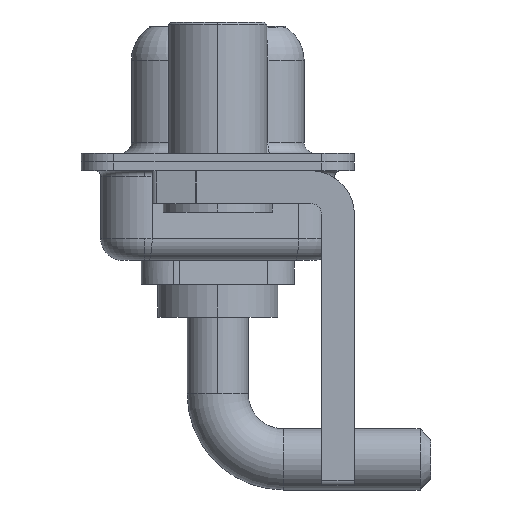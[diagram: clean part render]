
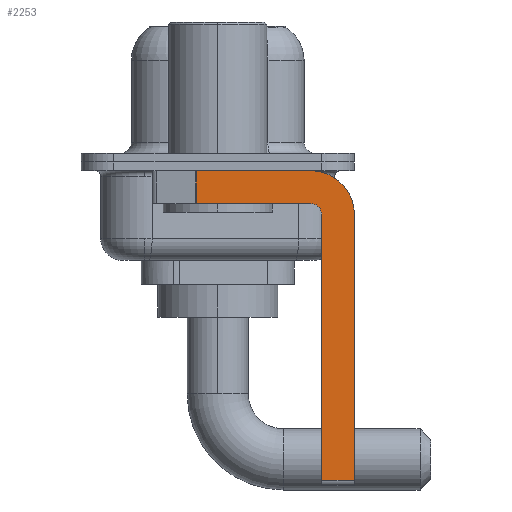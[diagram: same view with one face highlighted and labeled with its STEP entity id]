
A CAD part, left-side view. The second image highlights one B-rep face of the part: STEP entity #2253.
In plain terms, the highlighted planar face has unit normal (-1, 0, 0).
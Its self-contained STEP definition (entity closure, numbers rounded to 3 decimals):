
#216 = EDGE_LOOP ( 'NONE', ( #5971, #10110, #9486, #14276, #6099, #7282, #8405, #11327 ) ) ;
#619 = CARTESIAN_POINT ( 'NONE',  ( -2.9, 3., -0.4 ) ) ;
#848 = VERTEX_POINT ( 'NONE', #3708 ) ;
#1447 = LINE ( 'NONE', #4755, #10010 ) ;
#1519 = VECTOR ( 'NONE', #13532, 1000. ) ;
#1612 = VECTOR ( 'NONE', #6368, 1000. ) ;
#1747 = LINE ( 'NONE', #619, #13849 ) ;
#1781 = CARTESIAN_POINT ( 'NONE',  ( -2.9, -6.25, -2.4 ) ) ;
#2015 = CIRCLE ( 'NONE', #3934, 2. ) ;
#2098 = LINE ( 'NONE', #12490, #3447 ) ;
#2253 = ADVANCED_FACE ( 'NONE', ( #9279 ), #13863, .F. ) ;
#3018 = CARTESIAN_POINT ( 'NONE',  ( -2.9, -6.25, -14.55 ) ) ;
#3193 = CARTESIAN_POINT ( 'NONE',  ( -2.9, -4.25, -2.4 ) ) ;
#3383 = CARTESIAN_POINT ( 'NONE',  ( -2.9, 0.978, -1.9 ) ) ;
#3447 = VECTOR ( 'NONE', #7899, 1000. ) ;
#3708 = CARTESIAN_POINT ( 'NONE',  ( -2.9, 0.978, -0.4 ) ) ;
#3718 = VERTEX_POINT ( 'NONE', #3018 ) ;
#3934 = AXIS2_PLACEMENT_3D ( 'NONE', #7556, #10956, #8694 ) ;
#4465 = DIRECTION ( 'NONE',  ( 0., 0., 1. ) ) ;
#4477 = EDGE_CURVE ( 'NONE', #10130, #3718, #10084, .T. ) ;
#4755 = CARTESIAN_POINT ( 'NONE',  ( -2.9, -4.75, -14.8 ) ) ;
#4839 = AXIS2_PLACEMENT_3D ( 'NONE', #6173, #5333, #7453 ) ;
#5162 = LINE ( 'NONE', #1781, #1612 ) ;
#5333 = DIRECTION ( 'NONE',  ( 1., 0., 0. ) ) ;
#5971 = ORIENTED_EDGE ( 'NONE', *, *, #13015, .F. ) ;
#6003 = EDGE_CURVE ( 'NONE', #12529, #3718, #5162, .T. ) ;
#6099 = ORIENTED_EDGE ( 'NONE', *, *, #12725, .F. ) ;
#6173 = CARTESIAN_POINT ( 'NONE',  ( -2.9, -4.25, -2.4 ) ) ;
#6368 = DIRECTION ( 'NONE',  ( 0., 0., -1. ) ) ;
#6545 = VERTEX_POINT ( 'NONE', #14383 ) ;
#7081 = AXIS2_PLACEMENT_3D ( 'NONE', #3193, #11256, #4465 ) ;
#7282 = ORIENTED_EDGE ( 'NONE', *, *, #4477, .T. ) ;
#7453 = DIRECTION ( 'NONE',  ( 0., 0., -1. ) ) ;
#7537 = VERTEX_POINT ( 'NONE', #13275 ) ;
#7556 = CARTESIAN_POINT ( 'NONE',  ( -2.9, -4.25, -2.4 ) ) ;
#7889 = VERTEX_POINT ( 'NONE', #9103 ) ;
#7899 = DIRECTION ( 'NONE',  ( 0., 1., 0. ) ) ;
#8007 = EDGE_CURVE ( 'NONE', #7889, #8033, #2098, .T. ) ;
#8033 = VERTEX_POINT ( 'NONE', #3383 ) ;
#8301 = DIRECTION ( 'NONE',  ( 0., 0., 1. ) ) ;
#8405 = ORIENTED_EDGE ( 'NONE', *, *, #6003, .F. ) ;
#8694 = DIRECTION ( 'NONE',  ( 0., 0., -1. ) ) ;
#8942 = CARTESIAN_POINT ( 'NONE',  ( -2.9, -4.25, -14.55 ) ) ;
#9042 = EDGE_CURVE ( 'NONE', #6545, #12529, #2015, .T. ) ;
#9103 = CARTESIAN_POINT ( 'NONE',  ( -2.9, -4.25, -1.9 ) ) ;
#9237 = EDGE_CURVE ( 'NONE', #7537, #7889, #12606, .T. ) ;
#9242 = CARTESIAN_POINT ( 'NONE',  ( -2.9, -4.75, -14.55 ) ) ;
#9279 = FACE_OUTER_BOUND ( 'NONE', #216, .T. ) ;
#9486 = ORIENTED_EDGE ( 'NONE', *, *, #8007, .F. ) ;
#9810 = DIRECTION ( 'NONE',  ( 0., -1., 0. ) ) ;
#10010 = VECTOR ( 'NONE', #8301, 1000. ) ;
#10049 = LINE ( 'NONE', #11869, #12636 ) ;
#10084 = LINE ( 'NONE', #8942, #1519 ) ;
#10110 = ORIENTED_EDGE ( 'NONE', *, *, #12375, .T. ) ;
#10130 = VERTEX_POINT ( 'NONE', #9242 ) ;
#10753 = DIRECTION ( 'NONE',  ( 0., 0., -1. ) ) ;
#10956 = DIRECTION ( 'NONE',  ( 1., 0., 0. ) ) ;
#11256 = DIRECTION ( 'NONE',  ( -1., 0., 0. ) ) ;
#11327 = ORIENTED_EDGE ( 'NONE', *, *, #9042, .F. ) ;
#11399 = CARTESIAN_POINT ( 'NONE',  ( -2.9, -6.25, -2.4 ) ) ;
#11869 = CARTESIAN_POINT ( 'NONE',  ( -2.9, 0.978, -1.9 ) ) ;
#12375 = EDGE_CURVE ( 'NONE', #848, #8033, #10049, .T. ) ;
#12490 = CARTESIAN_POINT ( 'NONE',  ( -2.9, -4.25, -1.9 ) ) ;
#12529 = VERTEX_POINT ( 'NONE', #11399 ) ;
#12606 = CIRCLE ( 'NONE', #7081, 0.5 ) ;
#12636 = VECTOR ( 'NONE', #10753, 1000. ) ;
#12725 = EDGE_CURVE ( 'NONE', #10130, #7537, #1447, .T. ) ;
#13015 = EDGE_CURVE ( 'NONE', #848, #6545, #1747, .T. ) ;
#13275 = CARTESIAN_POINT ( 'NONE',  ( -2.9, -4.75, -2.4 ) ) ;
#13532 = DIRECTION ( 'NONE',  ( 0., -1., 0. ) ) ;
#13849 = VECTOR ( 'NONE', #9810, 1000. ) ;
#13863 = PLANE ( 'NONE',  #4839 ) ;
#14276 = ORIENTED_EDGE ( 'NONE', *, *, #9237, .F. ) ;
#14383 = CARTESIAN_POINT ( 'NONE',  ( -2.9, -4.25, -0.4 ) ) ;
